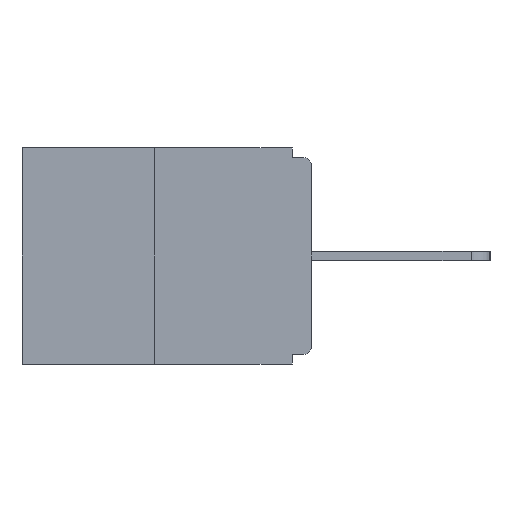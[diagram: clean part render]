
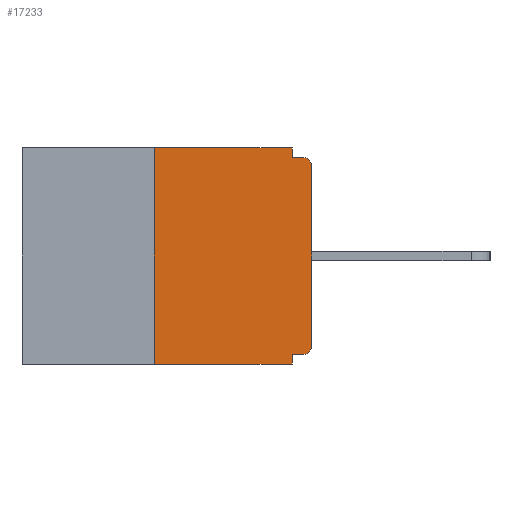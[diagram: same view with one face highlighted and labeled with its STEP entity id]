
A CAD part, left-side view. The second image highlights one B-rep face of the part: STEP entity #17233.
In plain terms, the highlighted planar face has unit normal (-1, 0, 0).
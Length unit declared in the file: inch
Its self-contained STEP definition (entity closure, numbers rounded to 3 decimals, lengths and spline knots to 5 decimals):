
#403 = ORIENTED_EDGE ( 'NONE', *, *, #12556, .F. ) ;
#417 = LINE ( 'NONE', #12462, #9206 ) ;
#471 = FACE_OUTER_BOUND ( 'NONE', #6239, .T. ) ;
#573 = AXIS2_PLACEMENT_3D ( 'NONE', #15128, #22085, #6503 ) ;
#898 = ORIENTED_EDGE ( 'NONE', *, *, #8317, .T. ) ;
#910 = LINE ( 'NONE', #7074, #4929 ) ;
#1078 = VERTEX_POINT ( 'NONE', #3179 ) ;
#1428 = EDGE_CURVE ( 'NONE', #7258, #1078, #21318, .T. ) ;
#2308 = CARTESIAN_POINT ( 'NONE',  ( 0., 0., -0.328 ) ) ;
#3179 = CARTESIAN_POINT ( 'NONE',  ( 0., 0.031, -0.343 ) ) ;
#3516 = LINE ( 'NONE', #11924, #12212 ) ;
#3714 = CIRCLE ( 'NONE', #16382, 0.015 ) ;
#4929 = VECTOR ( 'NONE', #5385, 39.37008 ) ;
#5248 = DIRECTION ( 'NONE',  ( 0., 0., -1. ) ) ;
#5385 = DIRECTION ( 'NONE',  ( 0., 0., 1. ) ) ;
#6171 = VERTEX_POINT ( 'NONE', #17467 ) ;
#6239 = EDGE_LOOP ( 'NONE', ( #403, #12827, #11391, #14150, #10313, #898, #15376, #15563, #21898, #17422 ) ) ;
#6328 = CARTESIAN_POINT ( 'NONE',  ( 0., 0.46, 0. ) ) ;
#6503 = DIRECTION ( 'NONE',  ( 0., 0., -1. ) ) ;
#6740 = VECTOR ( 'NONE', #16681, 39.37008 ) ;
#7054 = PLANE ( 'NONE',  #10136 ) ;
#7074 = CARTESIAN_POINT ( 'NONE',  ( 0., 0., 0. ) ) ;
#7258 = VERTEX_POINT ( 'NONE', #8069 ) ;
#7560 = DIRECTION ( 'NONE',  ( 0., 0., -1. ) ) ;
#7581 = DIRECTION ( 'NONE',  ( 0., 0., 1. ) ) ;
#7740 = VERTEX_POINT ( 'NONE', #12481 ) ;
#8069 = CARTESIAN_POINT ( 'NONE',  ( 0., 0.25, -0.343 ) ) ;
#8089 = CARTESIAN_POINT ( 'NONE',  ( 0., 0., -0.313 ) ) ;
#8317 = EDGE_CURVE ( 'NONE', #14776, #15899, #3714, .T. ) ;
#8477 = DIRECTION ( 'NONE',  ( 0., 0., -1. ) ) ;
#8941 = DIRECTION ( 'NONE',  ( 0., -1., 0. ) ) ;
#9206 = VECTOR ( 'NONE', #18008, 39.37008 ) ;
#9339 = VERTEX_POINT ( 'NONE', #18664 ) ;
#9824 = EDGE_CURVE ( 'NONE', #7258, #12871, #12701, .T. ) ;
#10096 = LINE ( 'NONE', #6328, #6740 ) ;
#10136 = AXIS2_PLACEMENT_3D ( 'NONE', #15812, #13751, #5248 ) ;
#10313 = ORIENTED_EDGE ( 'NONE', *, *, #11640, .F. ) ;
#10359 = VECTOR ( 'NONE', #21078, 39.37008 ) ;
#11097 = VECTOR ( 'NONE', #11867, 39.37008 ) ;
#11391 = ORIENTED_EDGE ( 'NONE', *, *, #1428, .T. ) ;
#11640 = EDGE_CURVE ( 'NONE', #14776, #13726, #14895, .T. ) ;
#11867 = DIRECTION ( 'NONE',  ( 0., 1., 0. ) ) ;
#11924 = CARTESIAN_POINT ( 'NONE',  ( 0., 0.031, -0.343 ) ) ;
#12212 = VECTOR ( 'NONE', #8477, 39.37008 ) ;
#12462 = CARTESIAN_POINT ( 'NONE',  ( 0., 0., -0.015 ) ) ;
#12481 = CARTESIAN_POINT ( 'NONE',  ( 0., 0.031, 0. ) ) ;
#12556 = EDGE_CURVE ( 'NONE', #12871, #7740, #10096, .T. ) ;
#12662 = EDGE_CURVE ( 'NONE', #13726, #1078, #3516, .T. ) ;
#12701 = LINE ( 'NONE', #21105, #14965 ) ;
#12827 = ORIENTED_EDGE ( 'NONE', *, *, #9824, .F. ) ;
#12871 = VERTEX_POINT ( 'NONE', #19295 ) ;
#12897 = DIRECTION ( 'NONE',  ( -1., 0., 0. ) ) ;
#13260 = CARTESIAN_POINT ( 'NONE',  ( 0., 0.031, -0.015 ) ) ;
#13600 = EDGE_CURVE ( 'NONE', #9339, #6171, #21964, .T. ) ;
#13726 = VERTEX_POINT ( 'NONE', #20816 ) ;
#13751 = DIRECTION ( 'NONE',  ( 1., 0., 0. ) ) ;
#14146 = LINE ( 'NONE', #21305, #10359 ) ;
#14150 = ORIENTED_EDGE ( 'NONE', *, *, #12662, .F. ) ;
#14460 = VERTEX_POINT ( 'NONE', #13260 ) ;
#14776 = VERTEX_POINT ( 'NONE', #21932 ) ;
#14895 = LINE ( 'NONE', #2308, #11097 ) ;
#14965 = VECTOR ( 'NONE', #7581, 39.37008 ) ;
#15128 = CARTESIAN_POINT ( 'NONE',  ( 0., 0.015, -0.03 ) ) ;
#15376 = ORIENTED_EDGE ( 'NONE', *, *, #19983, .T. ) ;
#15563 = ORIENTED_EDGE ( 'NONE', *, *, #13600, .T. ) ;
#15812 = CARTESIAN_POINT ( 'NONE',  ( 0., 0.46, 0. ) ) ;
#15899 = VERTEX_POINT ( 'NONE', #8089 ) ;
#16382 = AXIS2_PLACEMENT_3D ( 'NONE', #19825, #12897, #7560 ) ;
#16681 = DIRECTION ( 'NONE',  ( 0., -1., 0. ) ) ;
#17233 = ADVANCED_FACE ( 'NONE', ( #471 ), #7054, .F. ) ;
#17422 = ORIENTED_EDGE ( 'NONE', *, *, #19656, .F. ) ;
#17467 = CARTESIAN_POINT ( 'NONE',  ( 0., 0.015, -0.015 ) ) ;
#18008 = DIRECTION ( 'NONE',  ( 0., -1., 0. ) ) ;
#18242 = EDGE_CURVE ( 'NONE', #14460, #6171, #417, .T. ) ;
#18664 = CARTESIAN_POINT ( 'NONE',  ( 0., 0., -0.03 ) ) ;
#19295 = CARTESIAN_POINT ( 'NONE',  ( 0., 0.25, 0. ) ) ;
#19656 = EDGE_CURVE ( 'NONE', #7740, #14460, #14146, .T. ) ;
#19707 = CARTESIAN_POINT ( 'NONE',  ( 0., 0.46, -0.343 ) ) ;
#19825 = CARTESIAN_POINT ( 'NONE',  ( 0., 0.015, -0.313 ) ) ;
#19885 = VECTOR ( 'NONE', #8941, 39.37008 ) ;
#19983 = EDGE_CURVE ( 'NONE', #15899, #9339, #910, .T. ) ;
#20816 = CARTESIAN_POINT ( 'NONE',  ( 0., 0.031, -0.328 ) ) ;
#21078 = DIRECTION ( 'NONE',  ( 0., 0., -1. ) ) ;
#21105 = CARTESIAN_POINT ( 'NONE',  ( 0., 0.25, 0. ) ) ;
#21305 = CARTESIAN_POINT ( 'NONE',  ( 0., 0.031, 0. ) ) ;
#21318 = LINE ( 'NONE', #19707, #19885 ) ;
#21898 = ORIENTED_EDGE ( 'NONE', *, *, #18242, .F. ) ;
#21932 = CARTESIAN_POINT ( 'NONE',  ( 0., 0.015, -0.328 ) ) ;
#21964 = CIRCLE ( 'NONE', #573, 0.015 ) ;
#22085 = DIRECTION ( 'NONE',  ( -1., 0., 0. ) ) ;
